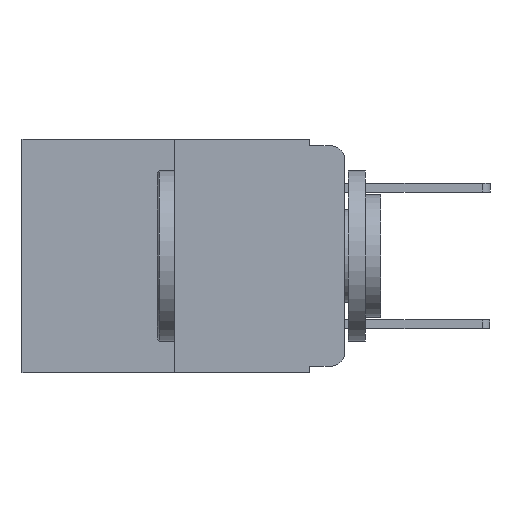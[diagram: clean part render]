
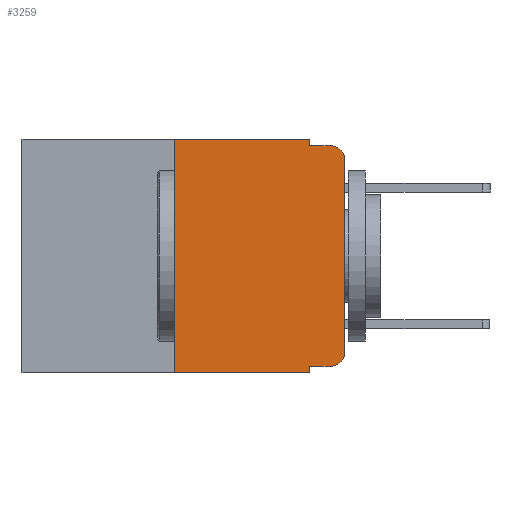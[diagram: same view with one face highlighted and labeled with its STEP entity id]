
A CAD part, left-side view. The second image highlights one B-rep face of the part: STEP entity #3259.
In plain terms, the highlighted planar face has unit normal (-1, 0, 0).
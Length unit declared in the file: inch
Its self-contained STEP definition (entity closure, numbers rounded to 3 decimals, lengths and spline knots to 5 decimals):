
#292 = ORIENTED_EDGE ( 'NONE', *, *, #6801, .T. ) ;
#436 = ORIENTED_EDGE ( 'NONE', *, *, #13756, .T. ) ;
#975 = DIRECTION ( 'NONE',  ( 0., -1., 0. ) ) ;
#1170 = LINE ( 'NONE', #4037, #10033 ) ;
#1563 = ORIENTED_EDGE ( 'NONE', *, *, #12756, .T. ) ;
#1607 = VERTEX_POINT ( 'NONE', #13895 ) ;
#1795 = EDGE_CURVE ( 'NONE', #14197, #15155, #1170, .T. ) ;
#1923 = EDGE_CURVE ( 'NONE', #2844, #15155, #11671, .T. ) ;
#1940 = VECTOR ( 'NONE', #975, 39.37008 ) ;
#2176 = CARTESIAN_POINT ( 'NONE',  ( 0., 0.051, 0. ) ) ;
#2638 = VERTEX_POINT ( 'NONE', #2176 ) ;
#2808 = VECTOR ( 'NONE', #15681, 39.37008 ) ;
#2844 = VERTEX_POINT ( 'NONE', #5897 ) ;
#2991 = CARTESIAN_POINT ( 'NONE',  ( 0., 0.25, 0. ) ) ;
#3006 = CARTESIAN_POINT ( 'NONE',  ( 0., 0.051, 0. ) ) ;
#3259 = ADVANCED_FACE ( 'NONE', ( #19846 ), #15453, .F. ) ;
#3500 = LINE ( 'NONE', #17518, #11627 ) ;
#3745 = VERTEX_POINT ( 'NONE', #9671 ) ;
#3964 = ORIENTED_EDGE ( 'NONE', *, *, #10774, .F. ) ;
#3990 = DIRECTION ( 'NONE',  ( -1., 0., 0. ) ) ;
#4037 = CARTESIAN_POINT ( 'NONE',  ( 0., 0.473, -0.343 ) ) ;
#4176 = ORIENTED_EDGE ( 'NONE', *, *, #9715, .F. ) ;
#4191 = DIRECTION ( 'NONE',  ( 0., -1., 0. ) ) ;
#4229 = ORIENTED_EDGE ( 'NONE', *, *, #7132, .F. ) ;
#4460 = CARTESIAN_POINT ( 'NONE',  ( 0., 0.473, 0. ) ) ;
#5008 = DIRECTION ( 'NONE',  ( -1., 0., 0. ) ) ;
#5601 = AXIS2_PLACEMENT_3D ( 'NONE', #13563, #3990, #15073 ) ;
#5777 = ORIENTED_EDGE ( 'NONE', *, *, #6387, .F. ) ;
#5850 = ORIENTED_EDGE ( 'NONE', *, *, #1795, .T. ) ;
#5897 = CARTESIAN_POINT ( 'NONE',  ( 0., 0.051, -0.333 ) ) ;
#5917 = ORIENTED_EDGE ( 'NONE', *, *, #1923, .F. ) ;
#6077 = LINE ( 'NONE', #8287, #17008 ) ;
#6103 = DIRECTION ( 'NONE',  ( 1., 0., 0. ) ) ;
#6366 = LINE ( 'NONE', #7637, #1940 ) ;
#6387 = EDGE_CURVE ( 'NONE', #14197, #13316, #3500, .T. ) ;
#6614 = DIRECTION ( 'NONE',  ( 0., -1., 0. ) ) ;
#6618 = CARTESIAN_POINT ( 'NONE',  ( 0., 0.051, 0. ) ) ;
#6746 = CARTESIAN_POINT ( 'NONE',  ( 0., 0.25, -0.343 ) ) ;
#6801 = EDGE_CURVE ( 'NONE', #1607, #9139, #16101, .T. ) ;
#7132 = EDGE_CURVE ( 'NONE', #13316, #2638, #6077, .T. ) ;
#7637 = CARTESIAN_POINT ( 'NONE',  ( 0., 0.051, -0.01 ) ) ;
#8287 = CARTESIAN_POINT ( 'NONE',  ( 0., 0.473, 0. ) ) ;
#9139 = VERTEX_POINT ( 'NONE', #16842 ) ;
#9671 = CARTESIAN_POINT ( 'NONE',  ( 0., 0.02, -0.01 ) ) ;
#9715 = EDGE_CURVE ( 'NONE', #2638, #14833, #18875, .T. ) ;
#9843 = VERTEX_POINT ( 'NONE', #9937 ) ;
#9907 = LINE ( 'NONE', #10767, #13436 ) ;
#9937 = CARTESIAN_POINT ( 'NONE',  ( 0., 0., -0.03 ) ) ;
#10033 = VECTOR ( 'NONE', #17841, 39.37008 ) ;
#10127 = LINE ( 'NONE', #16592, #13645 ) ;
#10309 = ORIENTED_EDGE ( 'NONE', *, *, #13128, .T. ) ;
#10708 = CARTESIAN_POINT ( 'NONE',  ( 0., 0.051, -0.343 ) ) ;
#10767 = CARTESIAN_POINT ( 'NONE',  ( 0., 0.051, -0.333 ) ) ;
#10774 = EDGE_CURVE ( 'NONE', #14833, #3745, #6366, .T. ) ;
#11224 = VECTOR ( 'NONE', #17416, 39.37008 ) ;
#11568 = DIRECTION ( 'NONE',  ( 0., 0., -1. ) ) ;
#11627 = VECTOR ( 'NONE', #14527, 39.37008 ) ;
#11671 = LINE ( 'NONE', #6618, #11224 ) ;
#12039 = CIRCLE ( 'NONE', #16564, 0.02 ) ;
#12519 = AXIS2_PLACEMENT_3D ( 'NONE', #4460, #6103, #11568 ) ;
#12756 = EDGE_CURVE ( 'NONE', #9843, #3745, #12039, .T. ) ;
#13128 = EDGE_CURVE ( 'NONE', #2844, #1607, #9907, .T. ) ;
#13316 = VERTEX_POINT ( 'NONE', #2991 ) ;
#13436 = VECTOR ( 'NONE', #4191, 39.37008 ) ;
#13563 = CARTESIAN_POINT ( 'NONE',  ( 0., 0.02, -0.313 ) ) ;
#13645 = VECTOR ( 'NONE', #19475, 39.37008 ) ;
#13756 = EDGE_CURVE ( 'NONE', #9139, #9843, #10127, .T. ) ;
#13895 = CARTESIAN_POINT ( 'NONE',  ( 0., 0.02, -0.333 ) ) ;
#14197 = VERTEX_POINT ( 'NONE', #6746 ) ;
#14488 = CARTESIAN_POINT ( 'NONE',  ( 0., 0.02, -0.03 ) ) ;
#14527 = DIRECTION ( 'NONE',  ( 0., 0., 1. ) ) ;
#14833 = VERTEX_POINT ( 'NONE', #17432 ) ;
#15073 = DIRECTION ( 'NONE',  ( 0., 0., -1. ) ) ;
#15155 = VERTEX_POINT ( 'NONE', #10708 ) ;
#15453 = PLANE ( 'NONE',  #12519 ) ;
#15681 = DIRECTION ( 'NONE',  ( 0., 0., -1. ) ) ;
#16029 = DIRECTION ( 'NONE',  ( 0., 0., -1. ) ) ;
#16101 = CIRCLE ( 'NONE', #5601, 0.02 ) ;
#16361 = EDGE_LOOP ( 'NONE', ( #436, #1563, #3964, #4176, #4229, #5777, #5850, #5917, #10309, #292 ) ) ;
#16564 = AXIS2_PLACEMENT_3D ( 'NONE', #14488, #5008, #16029 ) ;
#16592 = CARTESIAN_POINT ( 'NONE',  ( 0., 0., 0. ) ) ;
#16842 = CARTESIAN_POINT ( 'NONE',  ( 0., 0., -0.313 ) ) ;
#17008 = VECTOR ( 'NONE', #6614, 39.37008 ) ;
#17416 = DIRECTION ( 'NONE',  ( 0., 0., -1. ) ) ;
#17432 = CARTESIAN_POINT ( 'NONE',  ( 0., 0.051, -0.01 ) ) ;
#17518 = CARTESIAN_POINT ( 'NONE',  ( 0., 0.25, 0. ) ) ;
#17841 = DIRECTION ( 'NONE',  ( 0., -1., 0. ) ) ;
#18875 = LINE ( 'NONE', #3006, #2808 ) ;
#19475 = DIRECTION ( 'NONE',  ( 0., 0., 1. ) ) ;
#19846 = FACE_OUTER_BOUND ( 'NONE', #16361, .T. ) ;
